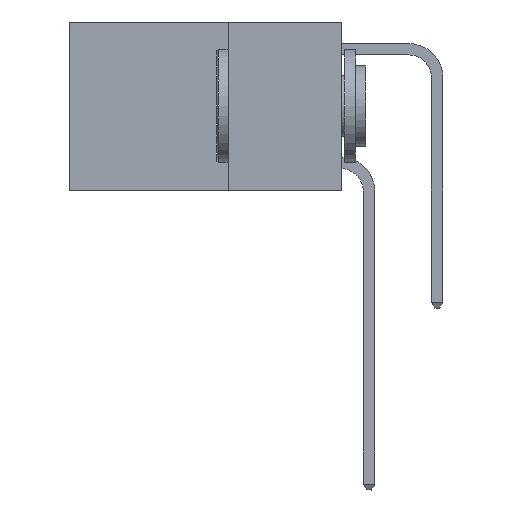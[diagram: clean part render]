
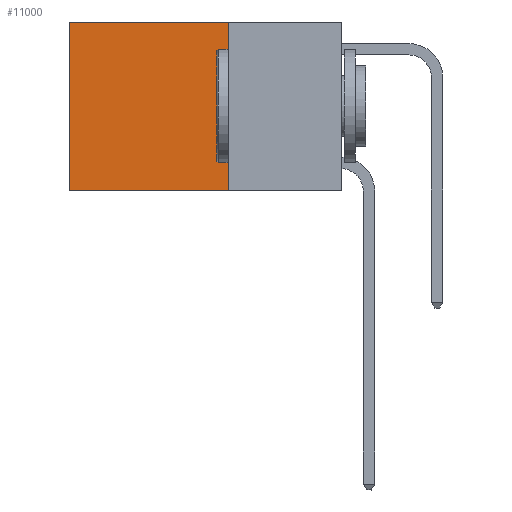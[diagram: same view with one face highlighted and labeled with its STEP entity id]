
A CAD part, left-side view. The second image highlights one B-rep face of the part: STEP entity #11000.
In plain terms, the highlighted planar face has unit normal (-1, 0, 0).
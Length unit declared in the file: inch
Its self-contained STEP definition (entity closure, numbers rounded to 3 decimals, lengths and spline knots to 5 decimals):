
#691 = DIRECTION ( 'NONE',  ( 0., 0., -1. ) ) ;
#785 = ORIENTED_EDGE ( 'NONE', *, *, #3317, .F. ) ;
#863 = CARTESIAN_POINT ( 'NONE',  ( 0.2625, 0.6, -0.37 ) ) ;
#2250 = ORIENTED_EDGE ( 'NONE', *, *, #3143, .F. ) ;
#3020 = LINE ( 'NONE', #9027, #11075 ) ;
#3143 = EDGE_CURVE ( 'NONE', #7981, #5673, #10311, .T. ) ;
#3317 = EDGE_CURVE ( 'NONE', #10469, #7981, #16215, .T. ) ;
#3761 = ORIENTED_EDGE ( 'NONE', *, *, #6952, .T. ) ;
#3871 = PLANE ( 'NONE',  #7470 ) ;
#4205 = DIRECTION ( 'NONE',  ( 0., 0., -1. ) ) ;
#5673 = VERTEX_POINT ( 'NONE', #863 ) ;
#6796 = VECTOR ( 'NONE', #17594, 39.37008 ) ;
#6952 = EDGE_CURVE ( 'NONE', #19928, #5673, #3020, .T. ) ;
#7008 = CARTESIAN_POINT ( 'NONE',  ( 0.2625, 0.25, 0. ) ) ;
#7264 = ORIENTED_EDGE ( 'NONE', *, *, #10118, .T. ) ;
#7470 = AXIS2_PLACEMENT_3D ( 'NONE', #7008, #10370, #691 ) ;
#7981 = VERTEX_POINT ( 'NONE', #10445 ) ;
#9027 = CARTESIAN_POINT ( 'NONE',  ( 0.2625, 0.6, 0. ) ) ;
#9458 = CARTESIAN_POINT ( 'NONE',  ( 0.2625, 0.25, 0. ) ) ;
#10118 = EDGE_CURVE ( 'NONE', #10469, #19928, #10933, .T. ) ;
#10311 = LINE ( 'NONE', #20275, #14562 ) ;
#10370 = DIRECTION ( 'NONE',  ( 1., 0., 0. ) ) ;
#10445 = CARTESIAN_POINT ( 'NONE',  ( 0.2625, 0.25, -0.37 ) ) ;
#10469 = VERTEX_POINT ( 'NONE', #12194 ) ;
#10933 = LINE ( 'NONE', #9458, #14672 ) ;
#10956 = DIRECTION ( 'NONE',  ( 0., 1., 0. ) ) ;
#11000 = ADVANCED_FACE ( 'NONE', ( #17527 ), #3871, .F. ) ;
#11075 = VECTOR ( 'NONE', #4205, 39.37008 ) ;
#12194 = CARTESIAN_POINT ( 'NONE',  ( 0.2625, 0.25, 0. ) ) ;
#12760 = EDGE_LOOP ( 'NONE', ( #3761, #2250, #785, #7264 ) ) ;
#12913 = CARTESIAN_POINT ( 'NONE',  ( 0.2625, 0.25, 0. ) ) ;
#14277 = DIRECTION ( 'NONE',  ( 0., 1., 0. ) ) ;
#14562 = VECTOR ( 'NONE', #10956, 39.37008 ) ;
#14672 = VECTOR ( 'NONE', #14277, 39.37008 ) ;
#15962 = CARTESIAN_POINT ( 'NONE',  ( 0.2625, 0.6, 0. ) ) ;
#16215 = LINE ( 'NONE', #12913, #6796 ) ;
#17527 = FACE_OUTER_BOUND ( 'NONE', #12760, .T. ) ;
#17594 = DIRECTION ( 'NONE',  ( 0., 0., -1. ) ) ;
#19928 = VERTEX_POINT ( 'NONE', #15962 ) ;
#20275 = CARTESIAN_POINT ( 'NONE',  ( 0.2625, 0.25, -0.37 ) ) ;
